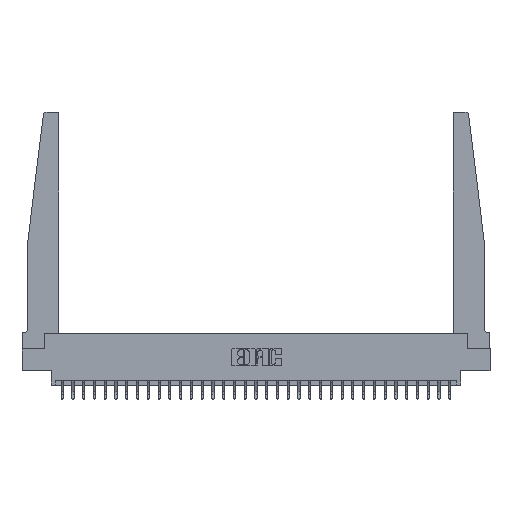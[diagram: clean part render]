
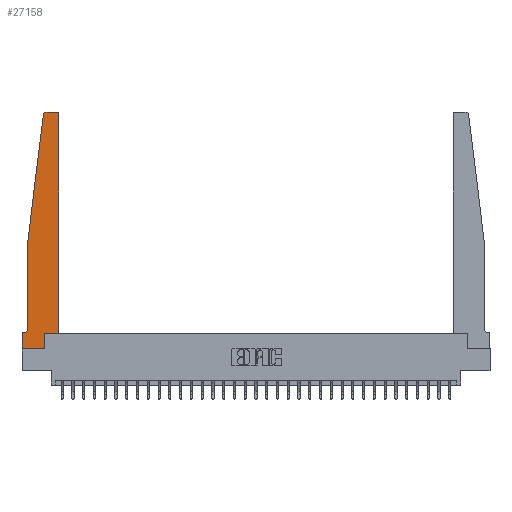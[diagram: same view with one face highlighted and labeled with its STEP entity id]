
A CAD part, top view. The second image highlights one B-rep face of the part: STEP entity #27158.
In plain terms, the highlighted planar face has unit normal (0, 0, 1).
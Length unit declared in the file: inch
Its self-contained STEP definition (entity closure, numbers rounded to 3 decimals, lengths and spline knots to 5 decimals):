
#236 = EDGE_LOOP ( 'NONE', ( #26210, #8317, #17365, #3940, #4094, #18393, #17950, #18944, #19267, #11332, #10469, #25306 ) ) ;
#399 = CARTESIAN_POINT ( 'NONE',  ( 0., 0.1875, 0.37 ) ) ;
#630 = VERTEX_POINT ( 'NONE', #1373 ) ;
#1148 = DIRECTION ( 'NONE',  ( -1., 0., 0. ) ) ;
#1373 = CARTESIAN_POINT ( 'NONE',  ( 0.065, 1.25, 0.37 ) ) ;
#1501 = VECTOR ( 'NONE', #18306, 39.37008 ) ;
#1588 = CARTESIAN_POINT ( 'NONE',  ( 0.425, 0.18, 0.37 ) ) ;
#1611 = CARTESIAN_POINT ( 'NONE',  ( 0.25, 2.75, 0.37 ) ) ;
#2206 = LINE ( 'NONE', #25634, #5445 ) ;
#2376 = LINE ( 'NONE', #1588, #20036 ) ;
#2474 = CARTESIAN_POINT ( 'NONE',  ( 0.425, 2.72, 0.37 ) ) ;
#3076 = DIRECTION ( 'NONE',  ( 1., 0., 0. ) ) ;
#3361 = CIRCLE ( 'NONE', #19164, 0.05 ) ;
#3714 = CARTESIAN_POINT ( 'NONE',  ( 0.27653, 2.72, 0.37 ) ) ;
#3787 = VERTEX_POINT ( 'NONE', #17890 ) ;
#3940 = ORIENTED_EDGE ( 'NONE', *, *, #10433, .T. ) ;
#4094 = ORIENTED_EDGE ( 'NONE', *, *, #9201, .T. ) ;
#4723 = CARTESIAN_POINT ( 'NONE',  ( 0.425, 0.18, 0.37 ) ) ;
#4925 = CARTESIAN_POINT ( 'NONE',  ( 0.395, 2.72, 0.37 ) ) ;
#5052 = CARTESIAN_POINT ( 'NONE',  ( 0., 0., 0.37 ) ) ;
#5260 = LINE ( 'NONE', #26402, #22979 ) ;
#5310 = VECTOR ( 'NONE', #12926, 39.37008 ) ;
#5445 = VECTOR ( 'NONE', #27993, 39.37008 ) ;
#5805 = VECTOR ( 'NONE', #21991, 39.37008 ) ;
#6018 = DIRECTION ( 'NONE',  ( 1., 0., 0. ) ) ;
#6388 = VECTOR ( 'NONE', #29758, 39.37008 ) ;
#6875 = CARTESIAN_POINT ( 'NONE',  ( 0., 0., 0.37 ) ) ;
#7186 = AXIS2_PLACEMENT_3D ( 'NONE', #3714, #19829, #6018 ) ;
#7247 = DIRECTION ( 'NONE',  ( 1., 0., 0. ) ) ;
#7686 = DIRECTION ( 'NONE',  ( 0., 0., -1. ) ) ;
#7737 = CARTESIAN_POINT ( 'NONE',  ( 0.395, 2.75, 0.37 ) ) ;
#8154 = CARTESIAN_POINT ( 'NONE',  ( 0.425, 0.18, 0.37 ) ) ;
#8317 = ORIENTED_EDGE ( 'NONE', *, *, #18400, .T. ) ;
#8918 = VERTEX_POINT ( 'NONE', #9036 ) ;
#9036 = CARTESIAN_POINT ( 'NONE',  ( 0.015, 0.1875, 0.37 ) ) ;
#9201 = EDGE_CURVE ( 'NONE', #14757, #8918, #3361, .T. ) ;
#9564 = EDGE_CURVE ( 'NONE', #27175, #11954, #17765, .T. ) ;
#10351 = EDGE_CURVE ( 'NONE', #17307, #630, #26095, .T. ) ;
#10433 = EDGE_CURVE ( 'NONE', #630, #14757, #2206, .T. ) ;
#10469 = ORIENTED_EDGE ( 'NONE', *, *, #23790, .T. ) ;
#10615 = CARTESIAN_POINT ( 'NONE',  ( 0.2605, 0.18, 0.37 ) ) ;
#10772 = LINE ( 'NONE', #10615, #5310 ) ;
#11332 = ORIENTED_EDGE ( 'NONE', *, *, #25394, .T. ) ;
#11530 = AXIS2_PLACEMENT_3D ( 'NONE', #4925, #21062, #7247 ) ;
#11715 = LINE ( 'NONE', #5052, #17101 ) ;
#11880 = VERTEX_POINT ( 'NONE', #399 ) ;
#11954 = VERTEX_POINT ( 'NONE', #28429 ) ;
#12246 = CIRCLE ( 'NONE', #11530, 0.03 ) ;
#12926 = DIRECTION ( 'NONE',  ( 0., 1., 0. ) ) ;
#12971 = CARTESIAN_POINT ( 'NONE',  ( 0.065, 0.2375, 0.37 ) ) ;
#13606 = EDGE_CURVE ( 'NONE', #29905, #3787, #10772, .T. ) ;
#13810 = EDGE_CURVE ( 'NONE', #23012, #29905, #29608, .T. ) ;
#14757 = VERTEX_POINT ( 'NONE', #12971 ) ;
#15195 = CARTESIAN_POINT ( 'NONE',  ( 0.2605, 0., 0.37 ) ) ;
#15271 = EDGE_CURVE ( 'NONE', #8918, #11880, #5260, .T. ) ;
#15384 = DIRECTION ( 'NONE',  ( 1., 0., 0. ) ) ;
#15521 = AXIS2_PLACEMENT_3D ( 'NONE', #23817, #16911, #3076 ) ;
#16646 = DIRECTION ( 'NONE',  ( 0., -1., 0. ) ) ;
#16911 = DIRECTION ( 'NONE',  ( 0., 0., 1. ) ) ;
#17101 = VECTOR ( 'NONE', #16646, 39.37008 ) ;
#17307 = VERTEX_POINT ( 'NONE', #20507 ) ;
#17347 = LINE ( 'NONE', #8154, #5805 ) ;
#17365 = ORIENTED_EDGE ( 'NONE', *, *, #10351, .T. ) ;
#17765 = LINE ( 'NONE', #1611, #29447 ) ;
#17770 = FACE_OUTER_BOUND ( 'NONE', #236, .T. ) ;
#17890 = CARTESIAN_POINT ( 'NONE',  ( 0.2605, 0.18, 0.37 ) ) ;
#17950 = ORIENTED_EDGE ( 'NONE', *, *, #26438, .T. ) ;
#18040 = CARTESIAN_POINT ( 'NONE',  ( 0., 0., 0.37 ) ) ;
#18306 = DIRECTION ( 'NONE',  ( -0.122, -0.992, 0. ) ) ;
#18393 = ORIENTED_EDGE ( 'NONE', *, *, #15271, .T. ) ;
#18400 = EDGE_CURVE ( 'NONE', #11954, #17307, #20554, .T. ) ;
#18944 = ORIENTED_EDGE ( 'NONE', *, *, #13810, .T. ) ;
#19164 = AXIS2_PLACEMENT_3D ( 'NONE', #21511, #7686, #23865 ) ;
#19267 = ORIENTED_EDGE ( 'NONE', *, *, #13606, .T. ) ;
#19829 = DIRECTION ( 'NONE',  ( 0., 0., 1. ) ) ;
#20028 = DIRECTION ( 'NONE',  ( -1., 0., 0. ) ) ;
#20036 = VECTOR ( 'NONE', #15384, 39.37008 ) ;
#20507 = CARTESIAN_POINT ( 'NONE',  ( 0.24675, 2.72367, 0.37 ) ) ;
#20554 = CIRCLE ( 'NONE', #7186, 0.03 ) ;
#21062 = DIRECTION ( 'NONE',  ( 0., 0., 1. ) ) ;
#21511 = CARTESIAN_POINT ( 'NONE',  ( 0.015, 0.2375, 0.37 ) ) ;
#21757 = VERTEX_POINT ( 'NONE', #4723 ) ;
#21991 = DIRECTION ( 'NONE',  ( 0., 1., 0. ) ) ;
#22979 = VECTOR ( 'NONE', #1148, 39.37008 ) ;
#23012 = VERTEX_POINT ( 'NONE', #6875 ) ;
#23790 = EDGE_CURVE ( 'NONE', #21757, #24105, #17347, .T. ) ;
#23817 = CARTESIAN_POINT ( 'NONE',  ( 0., 0.1875, 0.37 ) ) ;
#23865 = DIRECTION ( 'NONE',  ( -1., 0., 0. ) ) ;
#24105 = VERTEX_POINT ( 'NONE', #2474 ) ;
#25306 = ORIENTED_EDGE ( 'NONE', *, *, #29611, .T. ) ;
#25394 = EDGE_CURVE ( 'NONE', #3787, #21757, #2376, .T. ) ;
#25634 = CARTESIAN_POINT ( 'NONE',  ( 0.065, 1.25, 0.37 ) ) ;
#26095 = LINE ( 'NONE', #27691, #1501 ) ;
#26162 = PLANE ( 'NONE',  #15521 ) ;
#26210 = ORIENTED_EDGE ( 'NONE', *, *, #9564, .T. ) ;
#26402 = CARTESIAN_POINT ( 'NONE',  ( 0.065, 0.1875, 0.37 ) ) ;
#26438 = EDGE_CURVE ( 'NONE', #11880, #23012, #11715, .T. ) ;
#27158 = ADVANCED_FACE ( 'NONE', ( #17770 ), #26162, .T. ) ;
#27175 = VERTEX_POINT ( 'NONE', #7737 ) ;
#27691 = CARTESIAN_POINT ( 'NONE',  ( 0.065, 1.25, 0.37 ) ) ;
#27993 = DIRECTION ( 'NONE',  ( 0., -1., 0. ) ) ;
#28429 = CARTESIAN_POINT ( 'NONE',  ( 0.27653, 2.75, 0.37 ) ) ;
#29447 = VECTOR ( 'NONE', #20028, 39.37008 ) ;
#29608 = LINE ( 'NONE', #18040, #6388 ) ;
#29611 = EDGE_CURVE ( 'NONE', #24105, #27175, #12246, .T. ) ;
#29758 = DIRECTION ( 'NONE',  ( 1., 0., 0. ) ) ;
#29905 = VERTEX_POINT ( 'NONE', #15195 ) ;
